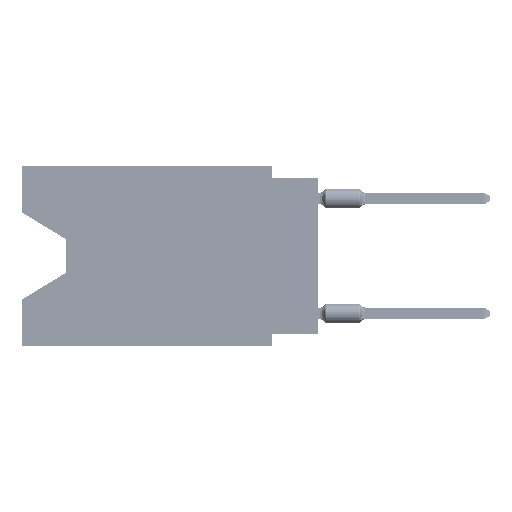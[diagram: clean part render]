
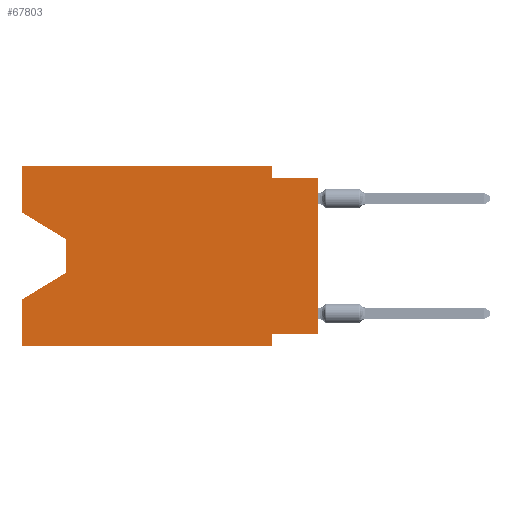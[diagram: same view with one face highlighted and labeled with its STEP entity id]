
A CAD part, left-side view. The second image highlights one B-rep face of the part: STEP entity #67803.
In plain terms, the highlighted planar face has unit normal (-1, 0, 0).
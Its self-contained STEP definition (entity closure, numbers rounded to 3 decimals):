
#514 = CARTESIAN_POINT ( 'NONE',  ( 0., 2.54, -9.271 ) ) ;
#802 = LINE ( 'NONE', #20286, #55061 ) ;
#1202 = CARTESIAN_POINT ( 'NONE',  ( 0., 16.383, -9.906 ) ) ;
#1447 = CARTESIAN_POINT ( 'NONE',  ( 0., 13.97, -5.893 ) ) ;
#1718 = ORIENTED_EDGE ( 'NONE', *, *, #9933, .T. ) ;
#1870 = CARTESIAN_POINT ( 'NONE',  ( 0., 16.383, 0. ) ) ;
#3041 = VERTEX_POINT ( 'NONE', #50745 ) ;
#3899 = CARTESIAN_POINT ( 'NONE',  ( 0., 2.54, -9.906 ) ) ;
#4505 = DIRECTION ( 'NONE',  ( 0., 0., 1. ) ) ;
#5857 = VECTOR ( 'NONE', #73635, 1000. ) ;
#6457 = ORIENTED_EDGE ( 'NONE', *, *, #17401, .F. ) ;
#6532 = VERTEX_POINT ( 'NONE', #10329 ) ;
#8294 = DIRECTION ( 'NONE',  ( 0., 0., 1. ) ) ;
#9108 = LINE ( 'NONE', #20491, #50941 ) ;
#9933 = EDGE_CURVE ( 'NONE', #23305, #52410, #19498, .T. ) ;
#10176 = LINE ( 'NONE', #46607, #58621 ) ;
#10329 = CARTESIAN_POINT ( 'NONE',  ( 0., 0., -9.271 ) ) ;
#10654 = VERTEX_POINT ( 'NONE', #37732 ) ;
#11819 = VERTEX_POINT ( 'NONE', #514 ) ;
#12976 = CARTESIAN_POINT ( 'NONE',  ( 0., 13.97, -4.013 ) ) ;
#13251 = LINE ( 'NONE', #24630, #26271 ) ;
#13936 = VERTEX_POINT ( 'NONE', #43016 ) ;
#14023 = CARTESIAN_POINT ( 'NONE',  ( 0., 16.383, 0. ) ) ;
#15709 = EDGE_CURVE ( 'NONE', #6532, #58406, #27600, .T. ) ;
#16196 = ORIENTED_EDGE ( 'NONE', *, *, #32781, .F. ) ;
#17154 = VECTOR ( 'NONE', #8294, 1000. ) ;
#17199 = LINE ( 'NONE', #3899, #20826 ) ;
#17401 = EDGE_CURVE ( 'NONE', #3041, #32735, #10176, .T. ) ;
#18087 = CARTESIAN_POINT ( 'NONE',  ( 0., 16.383, -2.546 ) ) ;
#19498 = LINE ( 'NONE', #61029, #60366 ) ;
#20187 = CARTESIAN_POINT ( 'NONE',  ( 0., 0., 0. ) ) ;
#20286 = CARTESIAN_POINT ( 'NONE',  ( 0., 13.97, -4.013 ) ) ;
#20411 = ORIENTED_EDGE ( 'NONE', *, *, #69802, .F. ) ;
#20491 = CARTESIAN_POINT ( 'NONE',  ( 0., 16.383, -9.906 ) ) ;
#20826 = VECTOR ( 'NONE', #27816, 1000. ) ;
#23305 = VERTEX_POINT ( 'NONE', #18087 ) ;
#24630 = CARTESIAN_POINT ( 'NONE',  ( 0., 13.97, -5.893 ) ) ;
#25465 = LINE ( 'NONE', #49351, #5857 ) ;
#25690 = VECTOR ( 'NONE', #25794, 1000. ) ;
#25794 = DIRECTION ( 'NONE',  ( 0., -1., 0. ) ) ;
#26271 = VECTOR ( 'NONE', #31688, 1000. ) ;
#26970 = ORIENTED_EDGE ( 'NONE', *, *, #69797, .F. ) ;
#27600 = LINE ( 'NONE', #20187, #55976 ) ;
#27816 = DIRECTION ( 'NONE',  ( 0., 0., -1. ) ) ;
#28934 = EDGE_CURVE ( 'NONE', #52410, #55817, #802, .T. ) ;
#29577 = ORIENTED_EDGE ( 'NONE', *, *, #40049, .T. ) ;
#31688 = DIRECTION ( 'NONE',  ( 0., 0.855, -0.519 ) ) ;
#31740 = DIRECTION ( 'NONE',  ( 0., 1., 0. ) ) ;
#31892 = ORIENTED_EDGE ( 'NONE', *, *, #28934, .T. ) ;
#32517 = LINE ( 'NONE', #50120, #42118 ) ;
#32735 = VERTEX_POINT ( 'NONE', #33156 ) ;
#32781 = EDGE_CURVE ( 'NONE', #23305, #61083, #63689, .T. ) ;
#33156 = CARTESIAN_POINT ( 'NONE',  ( 0., 2.54, -0.635 ) ) ;
#36609 = PLANE ( 'NONE',  #50367 ) ;
#36869 = DIRECTION ( 'NONE',  ( 0., 0., -1. ) ) ;
#37266 = EDGE_CURVE ( 'NONE', #11819, #10654, #17199, .T. ) ;
#37732 = CARTESIAN_POINT ( 'NONE',  ( 0., 2.54, -9.906 ) ) ;
#38862 = CARTESIAN_POINT ( 'NONE',  ( 0., 16.383, 0. ) ) ;
#40049 = EDGE_CURVE ( 'NONE', #55817, #13936, #13251, .T. ) ;
#40353 = DIRECTION ( 'NONE',  ( 0., 0., -1. ) ) ;
#42118 = VECTOR ( 'NONE', #31740, 1000. ) ;
#43016 = CARTESIAN_POINT ( 'NONE',  ( 0., 16.383, -7.36 ) ) ;
#44389 = DIRECTION ( 'NONE',  ( 0., -1., 0. ) ) ;
#45908 = CARTESIAN_POINT ( 'NONE',  ( 0., 0., -0.635 ) ) ;
#46545 = ORIENTED_EDGE ( 'NONE', *, *, #15709, .T. ) ;
#46607 = CARTESIAN_POINT ( 'NONE',  ( 0., 2.54, 0. ) ) ;
#47949 = VERTEX_POINT ( 'NONE', #1202 ) ;
#49351 = CARTESIAN_POINT ( 'NONE',  ( 0., 0., -0.635 ) ) ;
#50120 = CARTESIAN_POINT ( 'NONE',  ( 0., 0., -9.271 ) ) ;
#50367 = AXIS2_PLACEMENT_3D ( 'NONE', #54988, #73404, #61257 ) ;
#50745 = CARTESIAN_POINT ( 'NONE',  ( 0., 2.54, 0. ) ) ;
#50941 = VECTOR ( 'NONE', #44389, 1000. ) ;
#51110 = DIRECTION ( 'NONE',  ( 0., 0., 1. ) ) ;
#52410 = VERTEX_POINT ( 'NONE', #12976 ) ;
#54988 = CARTESIAN_POINT ( 'NONE',  ( 0., 16.383, 0. ) ) ;
#55061 = VECTOR ( 'NONE', #36869, 1000. ) ;
#55562 = EDGE_CURVE ( 'NONE', #47949, #13936, #75664, .T. ) ;
#55817 = VERTEX_POINT ( 'NONE', #1447 ) ;
#55976 = VECTOR ( 'NONE', #51110, 1000. ) ;
#56800 = VECTOR ( 'NONE', #4505, 1000. ) ;
#58193 = CARTESIAN_POINT ( 'NONE',  ( 0., 16.383, 0. ) ) ;
#58406 = VERTEX_POINT ( 'NONE', #45908 ) ;
#58621 = VECTOR ( 'NONE', #40353, 1000. ) ;
#59138 = ORIENTED_EDGE ( 'NONE', *, *, #55562, .F. ) ;
#60366 = VECTOR ( 'NONE', #73560, 1000. ) ;
#61029 = CARTESIAN_POINT ( 'NONE',  ( 0., 16.383, -2.546 ) ) ;
#61083 = VERTEX_POINT ( 'NONE', #14023 ) ;
#61170 = EDGE_LOOP ( 'NONE', ( #1718, #31892, #29577, #59138, #74504, #66001, #20411, #46545, #26970, #6457, #62231, #16196 ) ) ;
#61257 = DIRECTION ( 'NONE',  ( 0., 0., -1. ) ) ;
#61429 = LINE ( 'NONE', #1870, #25690 ) ;
#62042 = FACE_OUTER_BOUND ( 'NONE', #61170, .T. ) ;
#62231 = ORIENTED_EDGE ( 'NONE', *, *, #64668, .F. ) ;
#63689 = LINE ( 'NONE', #58193, #56800 ) ;
#64668 = EDGE_CURVE ( 'NONE', #61083, #3041, #61429, .T. ) ;
#66001 = ORIENTED_EDGE ( 'NONE', *, *, #37266, .F. ) ;
#66784 = EDGE_CURVE ( 'NONE', #47949, #10654, #9108, .T. ) ;
#67803 = ADVANCED_FACE ( 'NONE', ( #62042 ), #36609, .F. ) ;
#69797 = EDGE_CURVE ( 'NONE', #32735, #58406, #25465, .T. ) ;
#69802 = EDGE_CURVE ( 'NONE', #6532, #11819, #32517, .T. ) ;
#73404 = DIRECTION ( 'NONE',  ( 1., 0., 0. ) ) ;
#73560 = DIRECTION ( 'NONE',  ( 0., -0.855, -0.519 ) ) ;
#73635 = DIRECTION ( 'NONE',  ( 0., -1., 0. ) ) ;
#74504 = ORIENTED_EDGE ( 'NONE', *, *, #66784, .T. ) ;
#75664 = LINE ( 'NONE', #38862, #17154 ) ;
